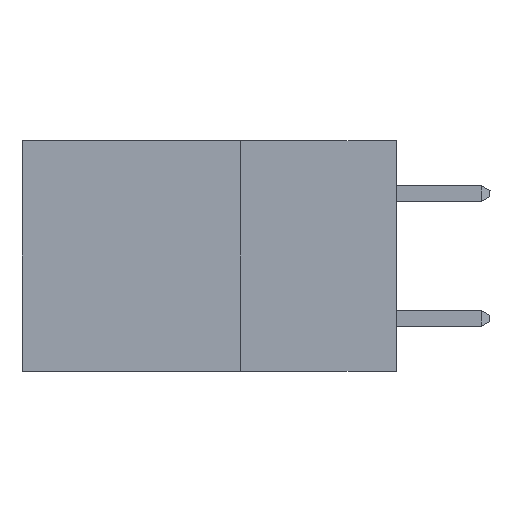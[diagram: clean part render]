
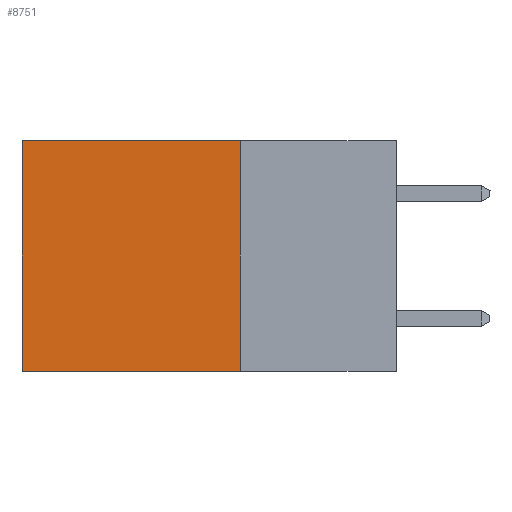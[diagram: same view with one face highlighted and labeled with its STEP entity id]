
A CAD part, left-side view. The second image highlights one B-rep face of the part: STEP entity #8751.
In plain terms, the highlighted planar face has unit normal (-1, 0, 0).
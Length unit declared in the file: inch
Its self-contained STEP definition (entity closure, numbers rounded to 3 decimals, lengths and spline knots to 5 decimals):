
#435 = ORIENTED_EDGE ( 'NONE', *, *, #6013, .F. ) ;
#833 = EDGE_CURVE ( 'NONE', #4516, #11775, #10640, .T. ) ;
#850 = EDGE_LOOP ( 'NONE', ( #4428, #435, #8316, #11139 ) ) ;
#1976 = DIRECTION ( 'NONE',  ( 0., 0., -1. ) ) ;
#2245 = LINE ( 'NONE', #5763, #11953 ) ;
#2322 = DIRECTION ( 'NONE',  ( 0., 1., 0. ) ) ;
#2608 = CARTESIAN_POINT ( 'NONE',  ( 0.298, 0.25, 0. ) ) ;
#2747 = DIRECTION ( 'NONE',  ( 0., 1., 0. ) ) ;
#3934 = EDGE_CURVE ( 'NONE', #4516, #8849, #8827, .T. ) ;
#3987 = VECTOR ( 'NONE', #2322, 39.37008 ) ;
#4428 = ORIENTED_EDGE ( 'NONE', *, *, #8183, .T. ) ;
#4439 = DIRECTION ( 'NONE',  ( 1., 0., 0. ) ) ;
#4516 = VERTEX_POINT ( 'NONE', #9835 ) ;
#5211 = CARTESIAN_POINT ( 'NONE',  ( 0.298, 0.6, -0.37 ) ) ;
#5339 = AXIS2_PLACEMENT_3D ( 'NONE', #11209, #4439, #11249 ) ;
#5763 = CARTESIAN_POINT ( 'NONE',  ( 0.298, 0.6, 0. ) ) ;
#6013 = EDGE_CURVE ( 'NONE', #8849, #11251, #12013, .T. ) ;
#6503 = CARTESIAN_POINT ( 'NONE',  ( 0.298, 0.25, -0.37 ) ) ;
#8183 = EDGE_CURVE ( 'NONE', #11775, #11251, #2245, .T. ) ;
#8316 = ORIENTED_EDGE ( 'NONE', *, *, #3934, .F. ) ;
#8385 = PLANE ( 'NONE',  #5339 ) ;
#8742 = CARTESIAN_POINT ( 'NONE',  ( 0.298, 0.25, 0. ) ) ;
#8751 = ADVANCED_FACE ( 'NONE', ( #10786 ), #8385, .F. ) ;
#8827 = LINE ( 'NONE', #2608, #11334 ) ;
#8849 = VERTEX_POINT ( 'NONE', #6503 ) ;
#9835 = CARTESIAN_POINT ( 'NONE',  ( 0.298, 0.25, 0. ) ) ;
#10548 = CARTESIAN_POINT ( 'NONE',  ( 0.298, 0.6, 0. ) ) ;
#10640 = LINE ( 'NONE', #8742, #12519 ) ;
#10786 = FACE_OUTER_BOUND ( 'NONE', #850, .T. ) ;
#11073 = CARTESIAN_POINT ( 'NONE',  ( 0.298, 0.25, -0.37 ) ) ;
#11139 = ORIENTED_EDGE ( 'NONE', *, *, #833, .T. ) ;
#11209 = CARTESIAN_POINT ( 'NONE',  ( 0.298, 0.25, 0. ) ) ;
#11249 = DIRECTION ( 'NONE',  ( 0., 0., -1. ) ) ;
#11251 = VERTEX_POINT ( 'NONE', #5211 ) ;
#11334 = VECTOR ( 'NONE', #1976, 39.37008 ) ;
#11576 = DIRECTION ( 'NONE',  ( 0., 0., -1. ) ) ;
#11775 = VERTEX_POINT ( 'NONE', #10548 ) ;
#11953 = VECTOR ( 'NONE', #11576, 39.37008 ) ;
#12013 = LINE ( 'NONE', #11073, #3987 ) ;
#12519 = VECTOR ( 'NONE', #2747, 39.37008 ) ;
